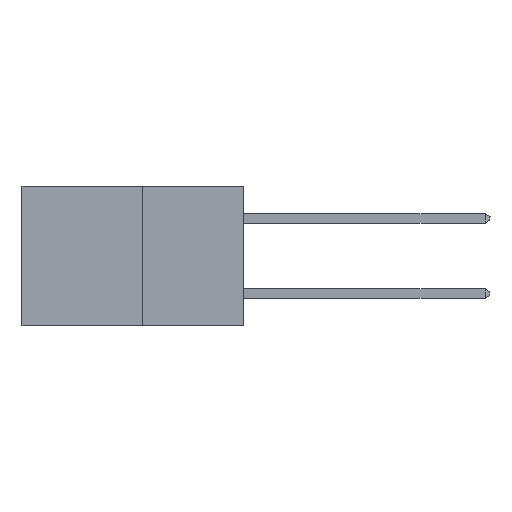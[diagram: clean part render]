
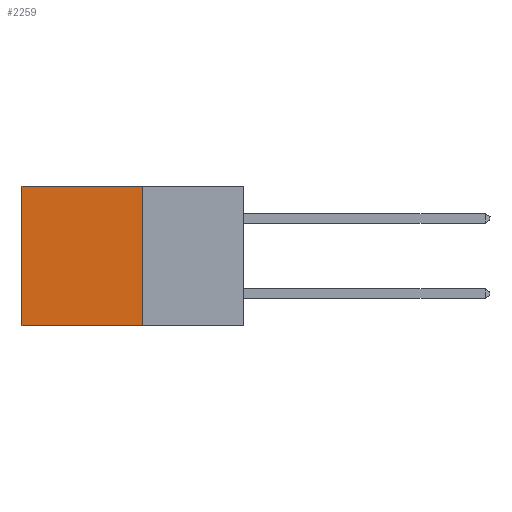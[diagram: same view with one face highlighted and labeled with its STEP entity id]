
A CAD part, left-side view. The second image highlights one B-rep face of the part: STEP entity #2259.
In plain terms, the highlighted planar face has unit normal (-1, 0, 0).
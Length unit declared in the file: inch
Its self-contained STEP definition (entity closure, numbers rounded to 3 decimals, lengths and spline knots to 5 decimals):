
#40 = VECTOR ( 'NONE', #621, 39.37008 ) ;
#43 = VERTEX_POINT ( 'NONE', #4395 ) ;
#315 = ORIENTED_EDGE ( 'NONE', *, *, #2036, .T. ) ;
#621 = DIRECTION ( 'NONE',  ( 0., 1., 0. ) ) ;
#788 = VECTOR ( 'NONE', #6582, 39.37008 ) ;
#810 = CARTESIAN_POINT ( 'NONE',  ( 0.277, 0.27, -0.37 ) ) ;
#967 = CARTESIAN_POINT ( 'NONE',  ( 0.277, 0.27, -0.37 ) ) ;
#971 = ORIENTED_EDGE ( 'NONE', *, *, #3502, .F. ) ;
#1512 = ORIENTED_EDGE ( 'NONE', *, *, #4082, .F. ) ;
#1672 = DIRECTION ( 'NONE',  ( 0., 0., -1. ) ) ;
#1848 = AXIS2_PLACEMENT_3D ( 'NONE', #967, #7503, #7489 ) ;
#2036 = EDGE_CURVE ( 'NONE', #3397, #6940, #6473, .T. ) ;
#2157 = FACE_OUTER_BOUND ( 'NONE', #6331, .T. ) ;
#2233 = VECTOR ( 'NONE', #1672, 39.37008 ) ;
#2259 = ADVANCED_FACE ( 'NONE', ( #2157 ), #2867, .F. ) ;
#2867 = PLANE ( 'NONE',  #1848 ) ;
#3220 = CARTESIAN_POINT ( 'NONE',  ( 0.277, 0.27, 0. ) ) ;
#3313 = VECTOR ( 'NONE', #6273, 39.37008 ) ;
#3397 = VERTEX_POINT ( 'NONE', #6953 ) ;
#3502 = EDGE_CURVE ( 'NONE', #6327, #43, #5922, .T. ) ;
#4068 = CARTESIAN_POINT ( 'NONE',  ( 0.277, 0.27, -0.37 ) ) ;
#4082 = EDGE_CURVE ( 'NONE', #43, #6940, #5459, .T. ) ;
#4231 = LINE ( 'NONE', #5435, #788 ) ;
#4395 = CARTESIAN_POINT ( 'NONE',  ( 0.277, 0.27, -0.37 ) ) ;
#5435 = CARTESIAN_POINT ( 'NONE',  ( 0.277, 0.27, 0. ) ) ;
#5459 = LINE ( 'NONE', #4068, #40 ) ;
#5788 = CARTESIAN_POINT ( 'NONE',  ( 0.277, 0.59, -0.37 ) ) ;
#5922 = LINE ( 'NONE', #810, #2233 ) ;
#6273 = DIRECTION ( 'NONE',  ( 0., 0., -1. ) ) ;
#6327 = VERTEX_POINT ( 'NONE', #3220 ) ;
#6331 = EDGE_LOOP ( 'NONE', ( #315, #1512, #971, #6690 ) ) ;
#6473 = LINE ( 'NONE', #6866, #3313 ) ;
#6582 = DIRECTION ( 'NONE',  ( 0., 1., 0. ) ) ;
#6690 = ORIENTED_EDGE ( 'NONE', *, *, #7865, .T. ) ;
#6866 = CARTESIAN_POINT ( 'NONE',  ( 0.277, 0.59, -0.37 ) ) ;
#6940 = VERTEX_POINT ( 'NONE', #5788 ) ;
#6953 = CARTESIAN_POINT ( 'NONE',  ( 0.277, 0.59, 0. ) ) ;
#7489 = DIRECTION ( 'NONE',  ( 0., 0., -1. ) ) ;
#7503 = DIRECTION ( 'NONE',  ( 1., 0., 0. ) ) ;
#7865 = EDGE_CURVE ( 'NONE', #6327, #3397, #4231, .T. ) ;
